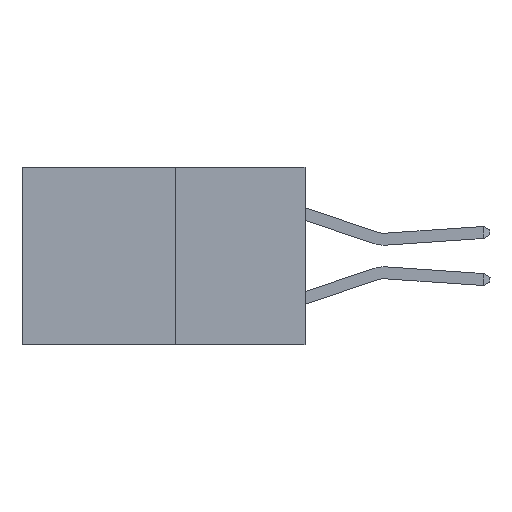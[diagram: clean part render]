
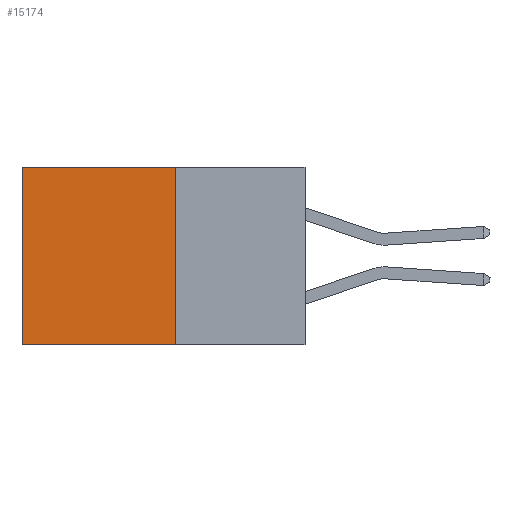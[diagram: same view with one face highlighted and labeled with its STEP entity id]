
A CAD part, left-side view. The second image highlights one B-rep face of the part: STEP entity #15174.
In plain terms, the highlighted planar face has unit normal (-1, 0, 0).
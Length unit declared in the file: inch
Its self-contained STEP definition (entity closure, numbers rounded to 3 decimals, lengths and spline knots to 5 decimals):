
#321 = VECTOR ( 'NONE', #7102, 39.37008 ) ;
#406 = VECTOR ( 'NONE', #20982, 39.37008 ) ;
#1931 = CARTESIAN_POINT ( 'NONE',  ( 0.277, 0.59, 0. ) ) ;
#1932 = DIRECTION ( 'NONE',  ( 0., 0., -1. ) ) ;
#2089 = CARTESIAN_POINT ( 'NONE',  ( 0.277, 0.59, -0.37 ) ) ;
#2507 = EDGE_CURVE ( 'NONE', #15906, #16005, #15330, .T. ) ;
#3208 = VECTOR ( 'NONE', #12093, 39.37008 ) ;
#3348 = ORIENTED_EDGE ( 'NONE', *, *, #20767, .F. ) ;
#3429 = DIRECTION ( 'NONE',  ( 0., 0., -1. ) ) ;
#6141 = VERTEX_POINT ( 'NONE', #12816 ) ;
#6780 = VERTEX_POINT ( 'NONE', #1931 ) ;
#7102 = DIRECTION ( 'NONE',  ( 0., 0., -1. ) ) ;
#7749 = LINE ( 'NONE', #2089, #16818 ) ;
#8327 = CARTESIAN_POINT ( 'NONE',  ( 0.277, 0.27, -0.37 ) ) ;
#8616 = CARTESIAN_POINT ( 'NONE',  ( 0.277, 0.27, -0.37 ) ) ;
#10030 = LINE ( 'NONE', #8327, #406 ) ;
#10431 = ORIENTED_EDGE ( 'NONE', *, *, #2507, .F. ) ;
#10633 = CARTESIAN_POINT ( 'NONE',  ( 0.277, 0.27, -0.37 ) ) ;
#10994 = CARTESIAN_POINT ( 'NONE',  ( 0.277, 0.27, -0.37 ) ) ;
#11390 = EDGE_CURVE ( 'NONE', #6780, #6141, #7749, .T. ) ;
#12093 = DIRECTION ( 'NONE',  ( 0., 1., 0. ) ) ;
#12451 = PLANE ( 'NONE',  #16046 ) ;
#12693 = ORIENTED_EDGE ( 'NONE', *, *, #11390, .T. ) ;
#12816 = CARTESIAN_POINT ( 'NONE',  ( 0.277, 0.59, -0.37 ) ) ;
#14263 = DIRECTION ( 'NONE',  ( 1., 0., 0. ) ) ;
#15174 = ADVANCED_FACE ( 'NONE', ( #23171 ), #12451, .F. ) ;
#15330 = LINE ( 'NONE', #8616, #321 ) ;
#15906 = VERTEX_POINT ( 'NONE', #16214 ) ;
#16005 = VERTEX_POINT ( 'NONE', #10994 ) ;
#16046 = AXIS2_PLACEMENT_3D ( 'NONE', #10633, #14263, #3429 ) ;
#16214 = CARTESIAN_POINT ( 'NONE',  ( 0.277, 0.27, 0. ) ) ;
#16379 = ORIENTED_EDGE ( 'NONE', *, *, #22262, .T. ) ;
#16818 = VECTOR ( 'NONE', #1932, 39.37008 ) ;
#16960 = EDGE_LOOP ( 'NONE', ( #12693, #3348, #10431, #16379 ) ) ;
#17082 = LINE ( 'NONE', #22907, #3208 ) ;
#20767 = EDGE_CURVE ( 'NONE', #16005, #6141, #10030, .T. ) ;
#20982 = DIRECTION ( 'NONE',  ( 0., 1., 0. ) ) ;
#22262 = EDGE_CURVE ( 'NONE', #15906, #6780, #17082, .T. ) ;
#22907 = CARTESIAN_POINT ( 'NONE',  ( 0.277, 0.27, 0. ) ) ;
#23171 = FACE_OUTER_BOUND ( 'NONE', #16960, .T. ) ;
